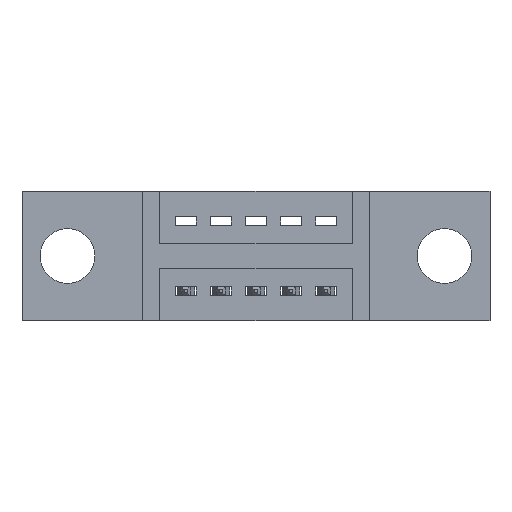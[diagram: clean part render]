
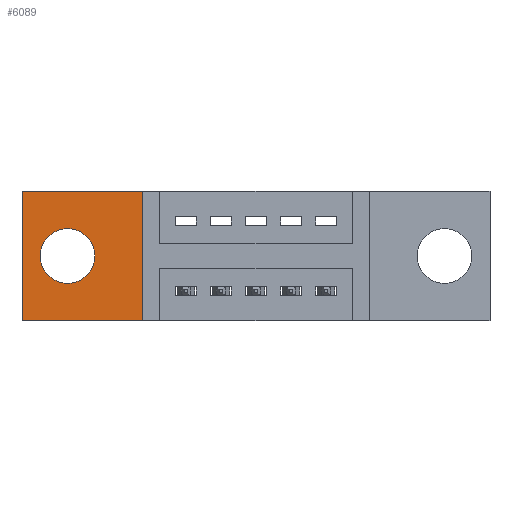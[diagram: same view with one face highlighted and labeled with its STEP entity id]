
A CAD part, front view. The second image highlights one B-rep face of the part: STEP entity #6089.
In plain terms, the highlighted planar face has unit normal (0, -1, 0).
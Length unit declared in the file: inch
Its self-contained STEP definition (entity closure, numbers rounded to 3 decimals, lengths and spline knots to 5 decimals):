
#574 = VECTOR ( 'NONE', #4179, 39.37008 ) ;
#579 = VERTEX_POINT ( 'NONE', #5014 ) ;
#746 = CARTESIAN_POINT ( 'NONE',  ( 0., 0.11, 0. ) ) ;
#1065 = DIRECTION ( 'NONE',  ( 0., -1., 0. ) ) ;
#1184 = CARTESIAN_POINT ( 'NONE',  ( 0., 0.11, 0. ) ) ;
#1609 = LINE ( 'NONE', #3458, #3134 ) ;
#2149 = ORIENTED_EDGE ( 'NONE', *, *, #6265, .F. ) ;
#2290 = CARTESIAN_POINT ( 'NONE',  ( 0.13, 0.11, -0.107 ) ) ;
#2318 = DIRECTION ( 'NONE',  ( 0., 0., 1. ) ) ;
#2385 = CARTESIAN_POINT ( 'NONE',  ( 0.13, 0.11, -0.263 ) ) ;
#2391 = CARTESIAN_POINT ( 'NONE',  ( 0., 0.11, -0.37 ) ) ;
#2433 = LINE ( 'NONE', #746, #574 ) ;
#2523 = DIRECTION ( 'NONE',  ( 0., -1., 0. ) ) ;
#2842 = DIRECTION ( 'NONE',  ( 0., 0., -1. ) ) ;
#3134 = VECTOR ( 'NONE', #6093, 39.37008 ) ;
#3154 = FACE_BOUND ( 'NONE', #7577, .T. ) ;
#3222 = CARTESIAN_POINT ( 'NONE',  ( 0., 0.11, -0.37 ) ) ;
#3458 = CARTESIAN_POINT ( 'NONE',  ( 0., 0.11, 0. ) ) ;
#3775 = VECTOR ( 'NONE', #4479, 39.37008 ) ;
#3902 = DIRECTION ( 'NONE',  ( 0., 0., -1. ) ) ;
#4101 = AXIS2_PLACEMENT_3D ( 'NONE', #3222, #2523, #3902 ) ;
#4179 = DIRECTION ( 'NONE',  ( 0., 0., -1. ) ) ;
#4251 = EDGE_CURVE ( 'NONE', #8870, #5461, #2433, .T. ) ;
#4479 = DIRECTION ( 'NONE',  ( 1., 0., 0. ) ) ;
#4496 = ORIENTED_EDGE ( 'NONE', *, *, #6316, .F. ) ;
#4724 = EDGE_LOOP ( 'NONE', ( #7795, #5688, #6039, #7958 ) ) ;
#4764 = VERTEX_POINT ( 'NONE', #4909 ) ;
#4909 = CARTESIAN_POINT ( 'NONE',  ( 0.3425, 0.11, -0.37 ) ) ;
#5014 = CARTESIAN_POINT ( 'NONE',  ( 0.3425, 0.11, 0. ) ) ;
#5052 = CARTESIAN_POINT ( 'NONE',  ( 0.3425, 0.11, 0. ) ) ;
#5130 = VERTEX_POINT ( 'NONE', #2385 ) ;
#5168 = PLANE ( 'NONE',  #4101 ) ;
#5380 = FACE_OUTER_BOUND ( 'NONE', #4724, .T. ) ;
#5461 = VERTEX_POINT ( 'NONE', #5809 ) ;
#5607 = CIRCLE ( 'NONE', #6568, 0.078 ) ;
#5662 = AXIS2_PLACEMENT_3D ( 'NONE', #7882, #1065, #5954 ) ;
#5688 = ORIENTED_EDGE ( 'NONE', *, *, #7108, .T. ) ;
#5809 = CARTESIAN_POINT ( 'NONE',  ( 0., 0.11, -0.37 ) ) ;
#5954 = DIRECTION ( 'NONE',  ( 0., 0., -1. ) ) ;
#6039 = ORIENTED_EDGE ( 'NONE', *, *, #8583, .T. ) ;
#6089 = ADVANCED_FACE ( 'NONE', ( #3154, #5380 ), #5168, .T. ) ;
#6093 = DIRECTION ( 'NONE',  ( -1., 0., 0. ) ) ;
#6265 = EDGE_CURVE ( 'NONE', #7589, #5130, #7521, .T. ) ;
#6307 = LINE ( 'NONE', #5052, #8674 ) ;
#6316 = EDGE_CURVE ( 'NONE', #5130, #7589, #5607, .T. ) ;
#6568 = AXIS2_PLACEMENT_3D ( 'NONE', #8758, #7459, #2842 ) ;
#6823 = EDGE_CURVE ( 'NONE', #579, #8870, #1609, .T. ) ;
#7108 = EDGE_CURVE ( 'NONE', #5461, #4764, #7516, .T. ) ;
#7459 = DIRECTION ( 'NONE',  ( 0., -1., 0. ) ) ;
#7516 = LINE ( 'NONE', #2391, #3775 ) ;
#7521 = CIRCLE ( 'NONE', #5662, 0.078 ) ;
#7577 = EDGE_LOOP ( 'NONE', ( #2149, #4496 ) ) ;
#7589 = VERTEX_POINT ( 'NONE', #2290 ) ;
#7795 = ORIENTED_EDGE ( 'NONE', *, *, #4251, .T. ) ;
#7882 = CARTESIAN_POINT ( 'NONE',  ( 0.13, 0.11, -0.185 ) ) ;
#7958 = ORIENTED_EDGE ( 'NONE', *, *, #6823, .T. ) ;
#8583 = EDGE_CURVE ( 'NONE', #4764, #579, #6307, .T. ) ;
#8674 = VECTOR ( 'NONE', #2318, 39.37008 ) ;
#8758 = CARTESIAN_POINT ( 'NONE',  ( 0.13, 0.11, -0.185 ) ) ;
#8870 = VERTEX_POINT ( 'NONE', #1184 ) ;
